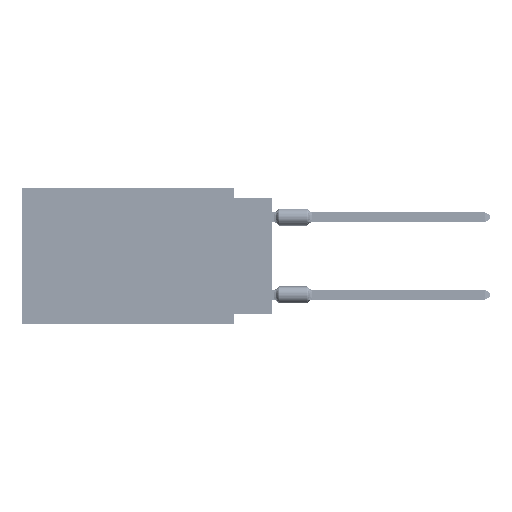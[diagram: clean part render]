
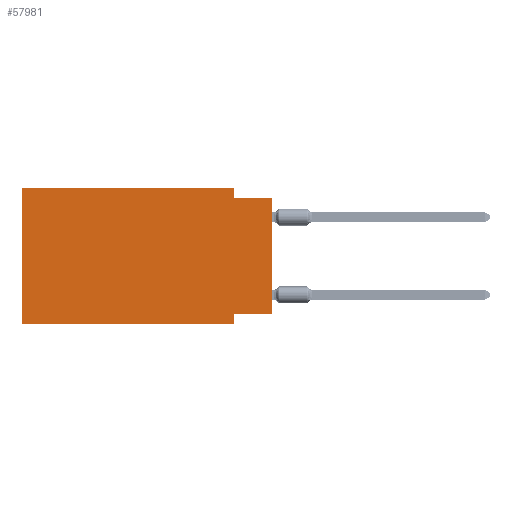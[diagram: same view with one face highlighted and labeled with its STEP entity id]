
A CAD part, left-side view. The second image highlights one B-rep face of the part: STEP entity #57981.
In plain terms, the highlighted planar face has unit normal (-1, 0, 0).
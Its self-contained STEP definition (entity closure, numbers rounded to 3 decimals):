
#895 = DIRECTION ( 'NONE',  ( 0., -1., 0. ) ) ;
#1426 = CARTESIAN_POINT ( 'NONE',  ( 0., 0., -8.255 ) ) ;
#2364 = CARTESIAN_POINT ( 'NONE',  ( 0., 16.383, 0. ) ) ;
#3448 = ORIENTED_EDGE ( 'NONE', *, *, #76992, .F. ) ;
#3830 = CARTESIAN_POINT ( 'NONE',  ( 0., 0., 0. ) ) ;
#6623 = DIRECTION ( 'NONE',  ( 0., -1., 0. ) ) ;
#9595 = CARTESIAN_POINT ( 'NONE',  ( 0., 2.54, -8.89 ) ) ;
#10635 = AXIS2_PLACEMENT_3D ( 'NONE', #22336, #54882, #41786 ) ;
#14670 = VERTEX_POINT ( 'NONE', #21587 ) ;
#15539 = CARTESIAN_POINT ( 'NONE',  ( 0., 0., -8.255 ) ) ;
#16358 = VECTOR ( 'NONE', #78183, 1000. ) ;
#16388 = EDGE_CURVE ( 'NONE', #48890, #40544, #30040, .T. ) ;
#18735 = EDGE_CURVE ( 'NONE', #14670, #85630, #74902, .T. ) ;
#20263 = DIRECTION ( 'NONE',  ( 0., -1., 0. ) ) ;
#21587 = CARTESIAN_POINT ( 'NONE',  ( 0., 16.383, -8.89 ) ) ;
#22269 = ORIENTED_EDGE ( 'NONE', *, *, #46059, .F. ) ;
#22336 = CARTESIAN_POINT ( 'NONE',  ( 0., 16.383, 0. ) ) ;
#22577 = VERTEX_POINT ( 'NONE', #51787 ) ;
#25314 = LINE ( 'NONE', #45634, #16358 ) ;
#30040 = LINE ( 'NONE', #3830, #83693 ) ;
#30726 = CARTESIAN_POINT ( 'NONE',  ( 0., 2.54, -8.89 ) ) ;
#30927 = DIRECTION ( 'NONE',  ( 0., 0., 1. ) ) ;
#35669 = VERTEX_POINT ( 'NONE', #74079 ) ;
#37793 = ORIENTED_EDGE ( 'NONE', *, *, #61170, .F. ) ;
#37883 = ORIENTED_EDGE ( 'NONE', *, *, #38576, .F. ) ;
#38576 = EDGE_CURVE ( 'NONE', #35669, #40544, #54501, .T. ) ;
#40467 = EDGE_CURVE ( 'NONE', #48890, #83435, #77405, .T. ) ;
#40544 = VERTEX_POINT ( 'NONE', #79621 ) ;
#41399 = CARTESIAN_POINT ( 'NONE',  ( 0., 0., -0.635 ) ) ;
#41786 = DIRECTION ( 'NONE',  ( 0., 0., -1. ) ) ;
#42007 = CARTESIAN_POINT ( 'NONE',  ( 0., 16.383, 0. ) ) ;
#43099 = DIRECTION ( 'NONE',  ( 0., 1., 0. ) ) ;
#43826 = ORIENTED_EDGE ( 'NONE', *, *, #16388, .T. ) ;
#43920 = LINE ( 'NONE', #9595, #52261 ) ;
#44222 = VECTOR ( 'NONE', #73997, 1000. ) ;
#45634 = CARTESIAN_POINT ( 'NONE',  ( 0., 16.383, 0. ) ) ;
#46059 = EDGE_CURVE ( 'NONE', #81497, #22577, #85629, .T. ) ;
#46447 = CARTESIAN_POINT ( 'NONE',  ( 0., 2.54, 0. ) ) ;
#48193 = VECTOR ( 'NONE', #6623, 1000. ) ;
#48549 = FACE_OUTER_BOUND ( 'NONE', #87393, .T. ) ;
#48890 = VERTEX_POINT ( 'NONE', #1426 ) ;
#49342 = VECTOR ( 'NONE', #20263, 1000. ) ;
#51617 = DIRECTION ( 'NONE',  ( 0., 0., -1. ) ) ;
#51787 = CARTESIAN_POINT ( 'NONE',  ( 0., 2.54, 0. ) ) ;
#52261 = VECTOR ( 'NONE', #51617, 1000. ) ;
#54501 = LINE ( 'NONE', #41399, #48193 ) ;
#54882 = DIRECTION ( 'NONE',  ( 1., 0., 0. ) ) ;
#57981 = ADVANCED_FACE ( 'NONE', ( #48549 ), #84197, .F. ) ;
#58791 = VECTOR ( 'NONE', #895, 1000. ) ;
#60900 = CARTESIAN_POINT ( 'NONE',  ( 0., 16.383, -8.89 ) ) ;
#61170 = EDGE_CURVE ( 'NONE', #22577, #35669, #80780, .T. ) ;
#61827 = VECTOR ( 'NONE', #43099, 1000. ) ;
#73997 = DIRECTION ( 'NONE',  ( 0., 0., -1. ) ) ;
#74079 = CARTESIAN_POINT ( 'NONE',  ( 0., 2.54, -0.635 ) ) ;
#74902 = LINE ( 'NONE', #60900, #49342 ) ;
#75344 = EDGE_CURVE ( 'NONE', #83435, #85630, #43920, .T. ) ;
#76992 = EDGE_CURVE ( 'NONE', #14670, #81497, #25314, .T. ) ;
#77405 = LINE ( 'NONE', #15539, #61827 ) ;
#77913 = CARTESIAN_POINT ( 'NONE',  ( 0., 2.54, -8.255 ) ) ;
#78183 = DIRECTION ( 'NONE',  ( 0., 0., 1. ) ) ;
#79621 = CARTESIAN_POINT ( 'NONE',  ( 0., 0., -0.635 ) ) ;
#79652 = ORIENTED_EDGE ( 'NONE', *, *, #75344, .F. ) ;
#80780 = LINE ( 'NONE', #46447, #44222 ) ;
#81497 = VERTEX_POINT ( 'NONE', #2364 ) ;
#83435 = VERTEX_POINT ( 'NONE', #77913 ) ;
#83693 = VECTOR ( 'NONE', #30927, 1000. ) ;
#84197 = PLANE ( 'NONE',  #10635 ) ;
#84811 = ORIENTED_EDGE ( 'NONE', *, *, #18735, .T. ) ;
#85629 = LINE ( 'NONE', #42007, #58791 ) ;
#85630 = VERTEX_POINT ( 'NONE', #30726 ) ;
#86822 = ORIENTED_EDGE ( 'NONE', *, *, #40467, .F. ) ;
#87393 = EDGE_LOOP ( 'NONE', ( #43826, #37883, #37793, #22269, #3448, #84811, #79652, #86822 ) ) ;
